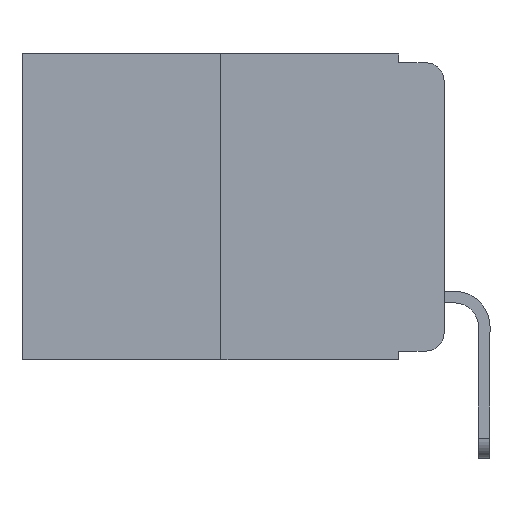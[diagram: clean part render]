
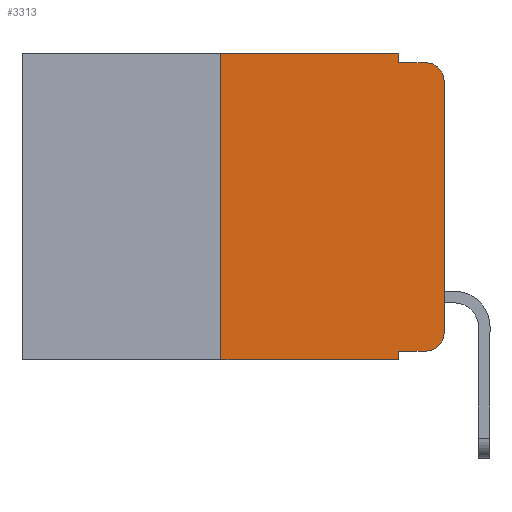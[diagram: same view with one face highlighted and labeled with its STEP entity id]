
A CAD part, left-side view. The second image highlights one B-rep face of the part: STEP entity #3313.
In plain terms, the highlighted planar face has unit normal (-1, 0, 0).
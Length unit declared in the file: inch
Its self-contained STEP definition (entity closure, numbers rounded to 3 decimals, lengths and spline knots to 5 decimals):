
#67 = VERTEX_POINT ( 'NONE', #21913 ) ;
#1211 = DIRECTION ( 'NONE',  ( -1., 0., 0. ) ) ;
#1442 = CARTESIAN_POINT ( 'NONE',  ( 0., 0.25, 0. ) ) ;
#1466 = EDGE_CURVE ( 'NONE', #16617, #14920, #17564, .T. ) ;
#1484 = EDGE_CURVE ( 'NONE', #5234, #16617, #21162, .T. ) ;
#2098 = ORIENTED_EDGE ( 'NONE', *, *, #2126, .T. ) ;
#2126 = EDGE_CURVE ( 'NONE', #11090, #5234, #11956, .T. ) ;
#3313 = ADVANCED_FACE ( 'NONE', ( #15952 ), #7764, .F. ) ;
#3537 = CARTESIAN_POINT ( 'NONE',  ( 0., 0.051, 0. ) ) ;
#4085 = LINE ( 'NONE', #1442, #7275 ) ;
#4353 = VECTOR ( 'NONE', #5408, 39.37008 ) ;
#4846 = ORIENTED_EDGE ( 'NONE', *, *, #19240, .F. ) ;
#4945 = LINE ( 'NONE', #3537, #4353 ) ;
#5234 = VERTEX_POINT ( 'NONE', #9233 ) ;
#5408 = DIRECTION ( 'NONE',  ( 0., 0., -1. ) ) ;
#7262 = CARTESIAN_POINT ( 'NONE',  ( 0., 0.051, -0.333 ) ) ;
#7275 = VECTOR ( 'NONE', #8959, 39.37008 ) ;
#7311 = VECTOR ( 'NONE', #8614, 39.37008 ) ;
#7341 = CARTESIAN_POINT ( 'NONE',  ( 0., 0.02, -0.01 ) ) ;
#7408 = DIRECTION ( 'NONE',  ( 1., 0., 0. ) ) ;
#7764 = PLANE ( 'NONE',  #20441 ) ;
#7926 = CARTESIAN_POINT ( 'NONE',  ( 0., 0.25, 0. ) ) ;
#7938 = EDGE_CURVE ( 'NONE', #14920, #18471, #19777, .T. ) ;
#8265 = ORIENTED_EDGE ( 'NONE', *, *, #1484, .T. ) ;
#8279 = VECTOR ( 'NONE', #22642, 39.37008 ) ;
#8614 = DIRECTION ( 'NONE',  ( 0., 0., -1. ) ) ;
#8715 = VECTOR ( 'NONE', #22032, 39.37008 ) ;
#8762 = CARTESIAN_POINT ( 'NONE',  ( 0., 0.051, -0.343 ) ) ;
#8909 = DIRECTION ( 'NONE',  ( 0., -1., 0. ) ) ;
#8959 = DIRECTION ( 'NONE',  ( 0., 0., 1. ) ) ;
#9221 = EDGE_CURVE ( 'NONE', #21752, #18471, #11834, .T. ) ;
#9233 = CARTESIAN_POINT ( 'NONE',  ( 0., 0.02, -0.333 ) ) ;
#9468 = CARTESIAN_POINT ( 'NONE',  ( 0., 0.02, -0.03 ) ) ;
#10926 = CARTESIAN_POINT ( 'NONE',  ( 0., 0.051, -0.01 ) ) ;
#11090 = VERTEX_POINT ( 'NONE', #7262 ) ;
#11148 = EDGE_CURVE ( 'NONE', #20185, #19831, #13140, .T. ) ;
#11291 = VECTOR ( 'NONE', #8909, 39.37008 ) ;
#11293 = DIRECTION ( 'NONE',  ( 0., 0., -1. ) ) ;
#11834 = LINE ( 'NONE', #19445, #11291 ) ;
#11956 = LINE ( 'NONE', #21193, #8279 ) ;
#12336 = CARTESIAN_POINT ( 'NONE',  ( 0., 0.02, -0.313 ) ) ;
#12429 = EDGE_LOOP ( 'NONE', ( #16300, #20656, #12708, #13832, #18487, #4846, #19484, #15490, #2098, #8265 ) ) ;
#12708 = ORIENTED_EDGE ( 'NONE', *, *, #9221, .F. ) ;
#13117 = CARTESIAN_POINT ( 'NONE',  ( 0., 0.473, -0.343 ) ) ;
#13140 = LINE ( 'NONE', #21104, #15643 ) ;
#13455 = VECTOR ( 'NONE', #21450, 39.37008 ) ;
#13832 = ORIENTED_EDGE ( 'NONE', *, *, #15108, .F. ) ;
#13920 = VERTEX_POINT ( 'NONE', #8762 ) ;
#14043 = CARTESIAN_POINT ( 'NONE',  ( 0., 0., 0. ) ) ;
#14766 = EDGE_CURVE ( 'NONE', #67, #13920, #22705, .T. ) ;
#14920 = VERTEX_POINT ( 'NONE', #17018 ) ;
#14924 = AXIS2_PLACEMENT_3D ( 'NONE', #12336, #1211, #17578 ) ;
#15108 = EDGE_CURVE ( 'NONE', #19831, #21752, #17313, .T. ) ;
#15490 = ORIENTED_EDGE ( 'NONE', *, *, #21711, .F. ) ;
#15643 = VECTOR ( 'NONE', #18012, 39.37008 ) ;
#15795 = CARTESIAN_POINT ( 'NONE',  ( 0., 0., -0.313 ) ) ;
#15952 = FACE_OUTER_BOUND ( 'NONE', #12429, .T. ) ;
#16300 = ORIENTED_EDGE ( 'NONE', *, *, #1466, .T. ) ;
#16617 = VERTEX_POINT ( 'NONE', #15795 ) ;
#17018 = CARTESIAN_POINT ( 'NONE',  ( 0., 0., -0.03 ) ) ;
#17313 = LINE ( 'NONE', #17455, #7311 ) ;
#17455 = CARTESIAN_POINT ( 'NONE',  ( 0., 0.051, 0. ) ) ;
#17564 = LINE ( 'NONE', #14043, #8715 ) ;
#17578 = DIRECTION ( 'NONE',  ( 0., 0., -1. ) ) ;
#17994 = DIRECTION ( 'NONE',  ( 0., 0., -1. ) ) ;
#18012 = DIRECTION ( 'NONE',  ( 0., -1., 0. ) ) ;
#18471 = VERTEX_POINT ( 'NONE', #7341 ) ;
#18487 = ORIENTED_EDGE ( 'NONE', *, *, #11148, .F. ) ;
#19240 = EDGE_CURVE ( 'NONE', #67, #20185, #4085, .T. ) ;
#19445 = CARTESIAN_POINT ( 'NONE',  ( 0., 0.051, -0.01 ) ) ;
#19484 = ORIENTED_EDGE ( 'NONE', *, *, #14766, .T. ) ;
#19726 = CARTESIAN_POINT ( 'NONE',  ( 0., 0.473, 0. ) ) ;
#19777 = CIRCLE ( 'NONE', #20753, 0.02 ) ;
#19831 = VERTEX_POINT ( 'NONE', #22911 ) ;
#20185 = VERTEX_POINT ( 'NONE', #7926 ) ;
#20441 = AXIS2_PLACEMENT_3D ( 'NONE', #19726, #7408, #17994 ) ;
#20656 = ORIENTED_EDGE ( 'NONE', *, *, #7938, .T. ) ;
#20753 = AXIS2_PLACEMENT_3D ( 'NONE', #9468, #21348, #11293 ) ;
#21104 = CARTESIAN_POINT ( 'NONE',  ( 0., 0.473, 0. ) ) ;
#21162 = CIRCLE ( 'NONE', #14924, 0.02 ) ;
#21193 = CARTESIAN_POINT ( 'NONE',  ( 0., 0.051, -0.333 ) ) ;
#21348 = DIRECTION ( 'NONE',  ( -1., 0., 0. ) ) ;
#21450 = DIRECTION ( 'NONE',  ( 0., -1., 0. ) ) ;
#21711 = EDGE_CURVE ( 'NONE', #11090, #13920, #4945, .T. ) ;
#21752 = VERTEX_POINT ( 'NONE', #10926 ) ;
#21913 = CARTESIAN_POINT ( 'NONE',  ( 0., 0.25, -0.343 ) ) ;
#22032 = DIRECTION ( 'NONE',  ( 0., 0., 1. ) ) ;
#22642 = DIRECTION ( 'NONE',  ( 0., -1., 0. ) ) ;
#22705 = LINE ( 'NONE', #13117, #13455 ) ;
#22911 = CARTESIAN_POINT ( 'NONE',  ( 0., 0.051, 0. ) ) ;
